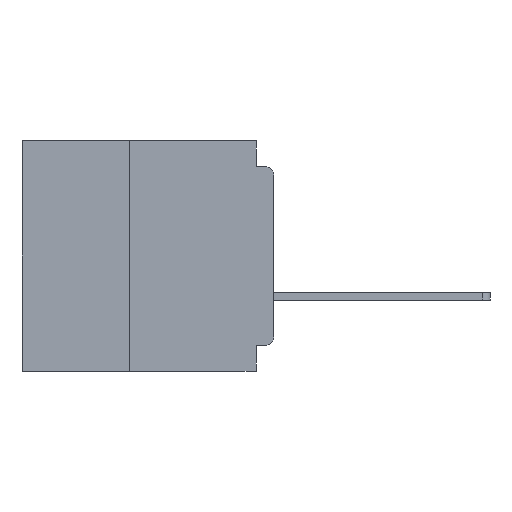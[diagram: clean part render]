
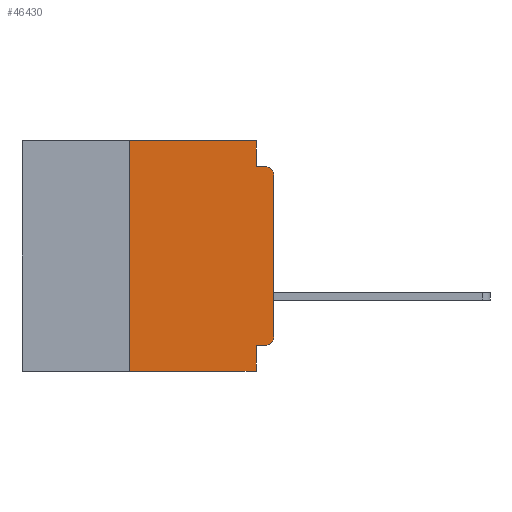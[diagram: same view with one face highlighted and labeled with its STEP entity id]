
A CAD part, left-side view. The second image highlights one B-rep face of the part: STEP entity #46430.
In plain terms, the highlighted planar face has unit normal (-1, 0, 0).
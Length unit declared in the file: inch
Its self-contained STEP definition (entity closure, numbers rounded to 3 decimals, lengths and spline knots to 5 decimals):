
#26 = LINE ( 'NONE', #31238, #26338 ) ;
#642 = PLANE ( 'NONE',  #63424 ) ;
#987 = VERTEX_POINT ( 'NONE', #22143 ) ;
#1077 = VERTEX_POINT ( 'NONE', #15006 ) ;
#1170 = VERTEX_POINT ( 'NONE', #10073 ) ;
#2052 = VERTEX_POINT ( 'NONE', #12712 ) ;
#3524 = EDGE_CURVE ( 'NONE', #39459, #57080, #6148, .T. ) ;
#3784 = ORIENTED_EDGE ( 'NONE', *, *, #18689, .F. ) ;
#3920 = DIRECTION ( 'NONE',  ( 0., 0., -1. ) ) ;
#4484 = VERTEX_POINT ( 'NONE', #49316 ) ;
#4526 = VECTOR ( 'NONE', #10383, 39.37008 ) ;
#5361 = ORIENTED_EDGE ( 'NONE', *, *, #41611, .T. ) ;
#5715 = CARTESIAN_POINT ( 'NONE',  ( 0., 0.437, 0. ) ) ;
#5932 = DIRECTION ( 'NONE',  ( 0., 0., -1. ) ) ;
#6148 = LINE ( 'NONE', #62376, #4526 ) ;
#8883 = VECTOR ( 'NONE', #9015, 39.37008 ) ;
#9015 = DIRECTION ( 'NONE',  ( 0., 1., 0. ) ) ;
#9262 = CARTESIAN_POINT ( 'NONE',  ( 0., 0.25, -0.4 ) ) ;
#9266 = DIRECTION ( 'NONE',  ( 0., 0., 1. ) ) ;
#10073 = CARTESIAN_POINT ( 'NONE',  ( 0., 0.031, -0.045 ) ) ;
#10095 = VECTOR ( 'NONE', #23931, 39.37008 ) ;
#10383 = DIRECTION ( 'NONE',  ( 0., 0., 1. ) ) ;
#12104 = DIRECTION ( 'NONE',  ( 0., 0., -1. ) ) ;
#12134 = EDGE_CURVE ( 'NONE', #987, #1077, #22826, .T. ) ;
#12712 = CARTESIAN_POINT ( 'NONE',  ( 0., 0.031, -0.4 ) ) ;
#13104 = ORIENTED_EDGE ( 'NONE', *, *, #12134, .F. ) ;
#14126 = CARTESIAN_POINT ( 'NONE',  ( 0., 0., -0.06 ) ) ;
#14304 = CARTESIAN_POINT ( 'NONE',  ( 0., 0.015, -0.06 ) ) ;
#14324 = AXIS2_PLACEMENT_3D ( 'NONE', #66367, #35331, #3920 ) ;
#15006 = CARTESIAN_POINT ( 'NONE',  ( 0., 0.031, -0.355 ) ) ;
#15682 = LINE ( 'NONE', #39980, #28001 ) ;
#17776 = EDGE_CURVE ( 'NONE', #29704, #31921, #24958, .T. ) ;
#17909 = CARTESIAN_POINT ( 'NONE',  ( 0., 0.031, 0. ) ) ;
#18634 = CARTESIAN_POINT ( 'NONE',  ( 0., 0.031, -0.4 ) ) ;
#18689 = EDGE_CURVE ( 'NONE', #28310, #1170, #49256, .T. ) ;
#18983 = AXIS2_PLACEMENT_3D ( 'NONE', #14304, #50818, #19591 ) ;
#19591 = DIRECTION ( 'NONE',  ( 0., 0., -1. ) ) ;
#19824 = CARTESIAN_POINT ( 'NONE',  ( 0., 0., 0. ) ) ;
#20641 = DIRECTION ( 'NONE',  ( 0., -1., 0. ) ) ;
#22143 = CARTESIAN_POINT ( 'NONE',  ( 0., 0.015, -0.355 ) ) ;
#22826 = LINE ( 'NONE', #24406, #8883 ) ;
#23931 = DIRECTION ( 'NONE',  ( 0., 0., -1. ) ) ;
#24406 = CARTESIAN_POINT ( 'NONE',  ( 0., 0., -0.355 ) ) ;
#24596 = ORIENTED_EDGE ( 'NONE', *, *, #38294, .F. ) ;
#24958 = CIRCLE ( 'NONE', #18983, 0.015 ) ;
#25246 = ORIENTED_EDGE ( 'NONE', *, *, #27920, .T. ) ;
#26071 = CARTESIAN_POINT ( 'NONE',  ( 0., 0.015, -0.045 ) ) ;
#26338 = VECTOR ( 'NONE', #20641, 39.37008 ) ;
#27920 = EDGE_CURVE ( 'NONE', #4484, #29704, #33166, .T. ) ;
#28001 = VECTOR ( 'NONE', #45192, 39.37008 ) ;
#28310 = VERTEX_POINT ( 'NONE', #17909 ) ;
#29677 = EDGE_CURVE ( 'NONE', #39459, #2052, #15682, .T. ) ;
#29704 = VERTEX_POINT ( 'NONE', #14126 ) ;
#31238 = CARTESIAN_POINT ( 'NONE',  ( 0., 0.437, 0. ) ) ;
#31921 = VERTEX_POINT ( 'NONE', #26071 ) ;
#32119 = CARTESIAN_POINT ( 'NONE',  ( 0., 0., -0.045 ) ) ;
#32387 = ORIENTED_EDGE ( 'NONE', *, *, #29677, .T. ) ;
#33007 = CARTESIAN_POINT ( 'NONE',  ( 0., 0.031, 0. ) ) ;
#33166 = LINE ( 'NONE', #19824, #60762 ) ;
#35331 = DIRECTION ( 'NONE',  ( -1., 0., 0. ) ) ;
#35461 = VECTOR ( 'NONE', #12104, 39.37008 ) ;
#37291 = DIRECTION ( 'NONE',  ( 1., 0., 0. ) ) ;
#37919 = LINE ( 'NONE', #18634, #10095 ) ;
#38294 = EDGE_CURVE ( 'NONE', #57080, #28310, #26, .T. ) ;
#38393 = EDGE_CURVE ( 'NONE', #1170, #31921, #47464, .T. ) ;
#39459 = VERTEX_POINT ( 'NONE', #9262 ) ;
#39876 = FACE_OUTER_BOUND ( 'NONE', #50788, .T. ) ;
#39980 = CARTESIAN_POINT ( 'NONE',  ( 0., 0.437, -0.4 ) ) ;
#41611 = EDGE_CURVE ( 'NONE', #987, #4484, #67167, .T. ) ;
#44746 = CARTESIAN_POINT ( 'NONE',  ( 0., 0.25, 0. ) ) ;
#45192 = DIRECTION ( 'NONE',  ( 0., -1., 0. ) ) ;
#46430 = ADVANCED_FACE ( 'NONE', ( #39876 ), #642, .F. ) ;
#47464 = LINE ( 'NONE', #32119, #59645 ) ;
#49256 = LINE ( 'NONE', #33007, #35461 ) ;
#49316 = CARTESIAN_POINT ( 'NONE',  ( 0., 0., -0.34 ) ) ;
#50788 = EDGE_LOOP ( 'NONE', ( #25246, #64943, #60402, #3784, #24596, #52827, #32387, #50801, #13104, #5361 ) ) ;
#50801 = ORIENTED_EDGE ( 'NONE', *, *, #63066, .F. ) ;
#50818 = DIRECTION ( 'NONE',  ( -1., 0., 0. ) ) ;
#52827 = ORIENTED_EDGE ( 'NONE', *, *, #3524, .F. ) ;
#57080 = VERTEX_POINT ( 'NONE', #44746 ) ;
#59645 = VECTOR ( 'NONE', #63223, 39.37008 ) ;
#60402 = ORIENTED_EDGE ( 'NONE', *, *, #38393, .F. ) ;
#60762 = VECTOR ( 'NONE', #9266, 39.37008 ) ;
#62376 = CARTESIAN_POINT ( 'NONE',  ( 0., 0.25, -0.4 ) ) ;
#63066 = EDGE_CURVE ( 'NONE', #1077, #2052, #37919, .T. ) ;
#63223 = DIRECTION ( 'NONE',  ( 0., -1., 0. ) ) ;
#63424 = AXIS2_PLACEMENT_3D ( 'NONE', #5715, #37291, #5932 ) ;
#64943 = ORIENTED_EDGE ( 'NONE', *, *, #17776, .T. ) ;
#66367 = CARTESIAN_POINT ( 'NONE',  ( 0., 0.015, -0.34 ) ) ;
#67167 = CIRCLE ( 'NONE', #14324, 0.015 ) ;
